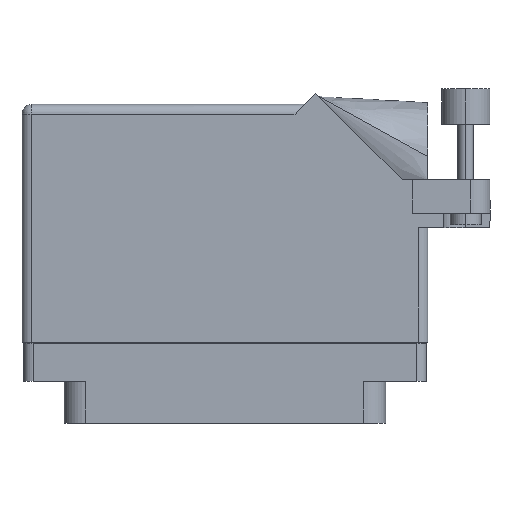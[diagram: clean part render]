
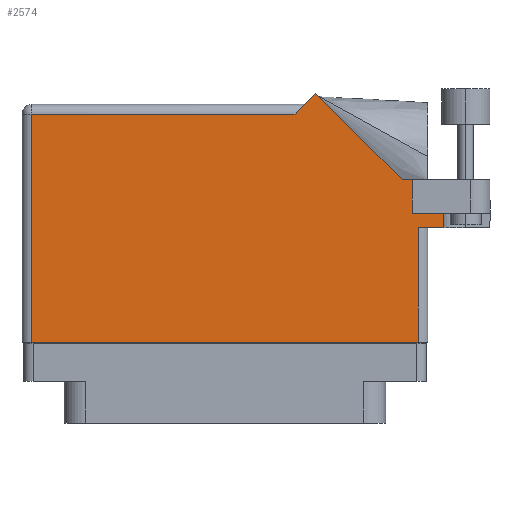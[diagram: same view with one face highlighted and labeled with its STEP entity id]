
A CAD part, front view. The second image highlights one B-rep face of the part: STEP entity #2574.
In plain terms, the highlighted face is planar.
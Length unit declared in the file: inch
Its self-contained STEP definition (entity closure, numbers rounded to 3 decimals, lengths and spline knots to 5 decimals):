
#333 = VERTEX_POINT ( 'NONE', #2644 ) ;
#537 = EDGE_CURVE ( 'NONE', #3558, #14688, #17369, .T. ) ;
#1621 = CARTESIAN_POINT ( 'NONE',  ( 1.244, 0.637, 0.455 ) ) ;
#2137 = VECTOR ( 'NONE', #8558, 39.37008 ) ;
#2205 = CARTESIAN_POINT ( 'NONE',  ( 1.244, -0.1, 0.455 ) ) ;
#2574 = ADVANCED_FACE ( 'NONE', ( #26980 ), #23282, .F. ) ;
#2644 = CARTESIAN_POINT ( 'NONE',  ( 0.58371, 1.50071, 0.455 ) ) ;
#2780 = VERTEX_POINT ( 'NONE', #45514 ) ;
#3288 = ORIENTED_EDGE ( 'NONE', *, *, #8944, .T. ) ;
#3558 = VERTEX_POINT ( 'NONE', #15788 ) ;
#3743 = ORIENTED_EDGE ( 'NONE', *, *, #537, .F. ) ;
#5312 = VERTEX_POINT ( 'NONE', #1621 ) ;
#5449 = VECTOR ( 'NONE', #34248, 39.37008 ) ;
#5801 = CARTESIAN_POINT ( 'NONE',  ( -1.244, 1.368, 0.455 ) ) ;
#6058 = DIRECTION ( 'NONE',  ( -0.707, 0.707, 0. ) ) ;
#6062 = CARTESIAN_POINT ( 'NONE',  ( 1.244, 0.637, 0.455 ) ) ;
#6123 = ORIENTED_EDGE ( 'NONE', *, *, #34961, .T. ) ;
#6640 = VERTEX_POINT ( 'NONE', #34332 ) ;
#6784 = LINE ( 'NONE', #28814, #42731 ) ;
#6923 = EDGE_CURVE ( 'NONE', #46573, #5312, #36582, .T. ) ;
#8558 = DIRECTION ( 'NONE',  ( -1., 0., 0. ) ) ;
#8723 = CARTESIAN_POINT ( 'NONE',  ( 1.706, 0.944, 0.455 ) ) ;
#8944 = EDGE_CURVE ( 'NONE', #5312, #14688, #31130, .T. ) ;
#10886 = DIRECTION ( 'NONE',  ( -1., 0., 0. ) ) ;
#10965 = DIRECTION ( 'NONE',  ( -1., 0., 0. ) ) ;
#10985 = EDGE_CURVE ( 'NONE', #2780, #333, #19336, .T. ) ;
#12203 = EDGE_CURVE ( 'NONE', #21967, #46573, #27325, .T. ) ;
#13000 = DIRECTION ( 'NONE',  ( 1., 0., 0. ) ) ;
#14688 = VERTEX_POINT ( 'NONE', #46765 ) ;
#14954 = EDGE_CURVE ( 'NONE', #30542, #31213, #29793, .T. ) ;
#15788 = CARTESIAN_POINT ( 'NONE',  ( 1.4075, 0.731, 0.455 ) ) ;
#16352 = VECTOR ( 'NONE', #17844, 39.37008 ) ;
#16767 = ORIENTED_EDGE ( 'NONE', *, *, #43035, .T. ) ;
#17217 = CARTESIAN_POINT ( 'NONE',  ( 1.206, 0.731, 0.455 ) ) ;
#17369 = LINE ( 'NONE', #30508, #5449 ) ;
#17844 = DIRECTION ( 'NONE',  ( 0., 1., 0. ) ) ;
#17863 = LINE ( 'NONE', #46033, #22885 ) ;
#17865 = EDGE_CURVE ( 'NONE', #52107, #6640, #17863, .T. ) ;
#19336 = LINE ( 'NONE', #50316, #38327 ) ;
#19379 = DIRECTION ( 'NONE',  ( 0., 0., -1. ) ) ;
#19631 = CARTESIAN_POINT ( 'NONE',  ( 1.206, 0.731, 0.455 ) ) ;
#21803 = DIRECTION ( 'NONE',  ( 0., 1., 0. ) ) ;
#21967 = VERTEX_POINT ( 'NONE', #47754 ) ;
#22683 = CARTESIAN_POINT ( 'NONE',  ( -1.306, 1.368, 0.455 ) ) ;
#22885 = VECTOR ( 'NONE', #21803, 39.37008 ) ;
#23074 = DIRECTION ( 'NONE',  ( 1., 0., 0. ) ) ;
#23282 = PLANE ( 'NONE',  #51922 ) ;
#23523 = VECTOR ( 'NONE', #13000, 39.37008 ) ;
#23715 = DIRECTION ( 'NONE',  ( 1., 0., 0. ) ) ;
#23795 = VECTOR ( 'NONE', #23715, 39.37008 ) ;
#25107 = EDGE_CURVE ( 'NONE', #52107, #3558, #49696, .T. ) ;
#25912 = ORIENTED_EDGE ( 'NONE', *, *, #12203, .T. ) ;
#25987 = DIRECTION ( 'NONE',  ( 0., -1., 0. ) ) ;
#26572 = CARTESIAN_POINT ( 'NONE',  ( -1.306, -0.1, 0.455 ) ) ;
#26980 = FACE_OUTER_BOUND ( 'NONE', #48159, .T. ) ;
#27325 = LINE ( 'NONE', #26572, #50170 ) ;
#28814 = CARTESIAN_POINT ( 'NONE',  ( -1.244, -0.1, 0.455 ) ) ;
#29790 = DIRECTION ( 'NONE',  ( -0.707, -0.707, 0. ) ) ;
#29793 = LINE ( 'NONE', #22683, #50020 ) ;
#30508 = CARTESIAN_POINT ( 'NONE',  ( 1.4075, 1.06177, 0.455 ) ) ;
#30542 = VERTEX_POINT ( 'NONE', #34623 ) ;
#30580 = ORIENTED_EDGE ( 'NONE', *, *, #31170, .T. ) ;
#30745 = ORIENTED_EDGE ( 'NONE', *, *, #10985, .T. ) ;
#30809 = ORIENTED_EDGE ( 'NONE', *, *, #6923, .T. ) ;
#31130 = LINE ( 'NONE', #32412, #23523 ) ;
#31170 = EDGE_CURVE ( 'NONE', #31213, #21967, #6784, .T. ) ;
#31213 = VERTEX_POINT ( 'NONE', #5801 ) ;
#32412 = CARTESIAN_POINT ( 'NONE',  ( 1.306, 0.637, 0.455 ) ) ;
#34248 = DIRECTION ( 'NONE',  ( 0., -1., 0. ) ) ;
#34315 = LINE ( 'NONE', #8723, #2137 ) ;
#34332 = CARTESIAN_POINT ( 'NONE',  ( 1.206, 0.944, 0.455 ) ) ;
#34623 = CARTESIAN_POINT ( 'NONE',  ( 0.451, 1.368, 0.455 ) ) ;
#34961 = EDGE_CURVE ( 'NONE', #333, #30542, #45424, .T. ) ;
#35145 = CARTESIAN_POINT ( 'NONE',  ( -1.306, 1.43, 0.455 ) ) ;
#36582 = LINE ( 'NONE', #6062, #16352 ) ;
#38327 = VECTOR ( 'NONE', #6058, 39.37008 ) ;
#41810 = CARTESIAN_POINT ( 'NONE',  ( 0.513, 1.43, 0.455 ) ) ;
#42731 = VECTOR ( 'NONE', #25987, 39.37008 ) ;
#43035 = EDGE_CURVE ( 'NONE', #6640, #2780, #34315, .T. ) ;
#44134 = VECTOR ( 'NONE', #29790, 39.37008 ) ;
#45424 = LINE ( 'NONE', #41810, #44134 ) ;
#45514 = CARTESIAN_POINT ( 'NONE',  ( 1.14042, 0.944, 0.455 ) ) ;
#45921 = ORIENTED_EDGE ( 'NONE', *, *, #25107, .F. ) ;
#46033 = CARTESIAN_POINT ( 'NONE',  ( 1.206, 0.731, 0.455 ) ) ;
#46573 = VERTEX_POINT ( 'NONE', #2205 ) ;
#46765 = CARTESIAN_POINT ( 'NONE',  ( 1.4075, 0.637, 0.455 ) ) ;
#47754 = CARTESIAN_POINT ( 'NONE',  ( -1.244, -0.1, 0.455 ) ) ;
#48159 = EDGE_LOOP ( 'NONE', ( #25912, #30809, #3288, #3743, #45921, #51479, #16767, #30745, #6123, #50384, #30580 ) ) ;
#49696 = LINE ( 'NONE', #19631, #23795 ) ;
#50020 = VECTOR ( 'NONE', #10886, 39.37008 ) ;
#50170 = VECTOR ( 'NONE', #23074, 39.37008 ) ;
#50316 = CARTESIAN_POINT ( 'NONE',  ( 1.14042, 0.944, 0.455 ) ) ;
#50384 = ORIENTED_EDGE ( 'NONE', *, *, #14954, .T. ) ;
#51479 = ORIENTED_EDGE ( 'NONE', *, *, #17865, .T. ) ;
#51922 = AXIS2_PLACEMENT_3D ( 'NONE', #35145, #19379, #10965 ) ;
#52107 = VERTEX_POINT ( 'NONE', #17217 ) ;
